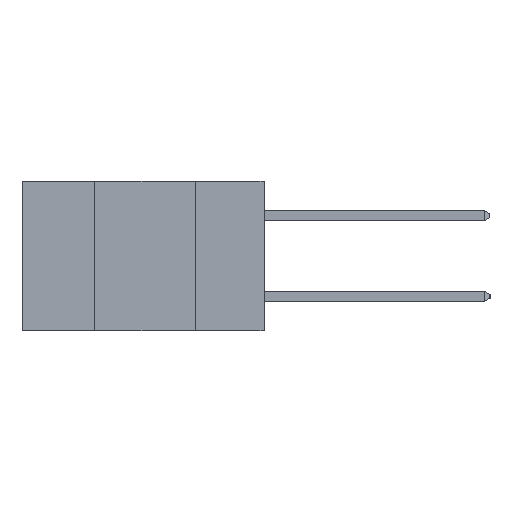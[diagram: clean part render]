
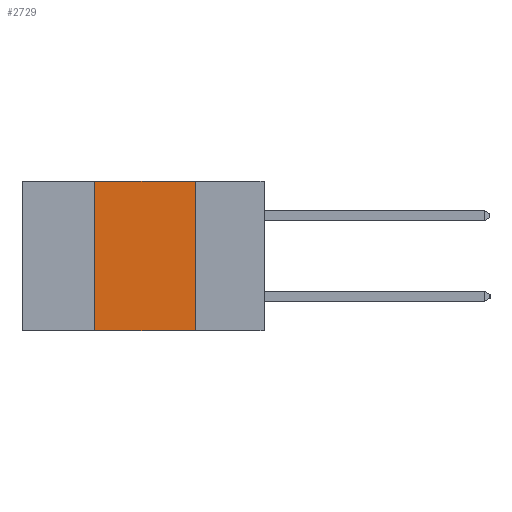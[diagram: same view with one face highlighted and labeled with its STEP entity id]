
A CAD part, left-side view. The second image highlights one B-rep face of the part: STEP entity #2729.
In plain terms, the highlighted planar face has unit normal (-1, 0, 0).
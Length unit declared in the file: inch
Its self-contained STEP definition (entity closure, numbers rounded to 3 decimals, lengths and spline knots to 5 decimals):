
#349 = DIRECTION ( 'NONE',  ( 0., -1., 0. ) ) ;
#1070 = EDGE_CURVE ( 'NONE', #13673, #6517, #11731, .T. ) ;
#2141 = ORIENTED_EDGE ( 'NONE', *, *, #1070, .F. ) ;
#2276 = CARTESIAN_POINT ( 'NONE',  ( 0., 0.17, -0.37 ) ) ;
#2729 = ADVANCED_FACE ( 'NONE', ( #12255 ), #10736, .F. ) ;
#3753 = LINE ( 'NONE', #13724, #12672 ) ;
#4193 = LINE ( 'NONE', #5024, #13782 ) ;
#4704 = EDGE_CURVE ( 'NONE', #12882, #13924, #4193, .T. ) ;
#4868 = VECTOR ( 'NONE', #349, 39.37008 ) ;
#4970 = DIRECTION ( 'NONE',  ( 0., -1., 0. ) ) ;
#5024 = CARTESIAN_POINT ( 'NONE',  ( 0., 0.6, -0.37 ) ) ;
#5704 = EDGE_CURVE ( 'NONE', #6517, #13924, #9442, .T. ) ;
#5843 = VECTOR ( 'NONE', #12835, 39.37008 ) ;
#6000 = CARTESIAN_POINT ( 'NONE',  ( 0., 0.42, -0.37 ) ) ;
#6517 = VERTEX_POINT ( 'NONE', #12447 ) ;
#7185 = ORIENTED_EDGE ( 'NONE', *, *, #5704, .F. ) ;
#7706 = CARTESIAN_POINT ( 'NONE',  ( 0., 0.42, 0. ) ) ;
#8224 = CARTESIAN_POINT ( 'NONE',  ( 0., 0.6, 0. ) ) ;
#9442 = LINE ( 'NONE', #12552, #5843 ) ;
#10076 = EDGE_LOOP ( 'NONE', ( #7185, #2141, #11559, #13896 ) ) ;
#10690 = CARTESIAN_POINT ( 'NONE',  ( 0., 0.6, 0. ) ) ;
#10736 = PLANE ( 'NONE',  #15499 ) ;
#10807 = DIRECTION ( 'NONE',  ( 1., 0., 0. ) ) ;
#10990 = DIRECTION ( 'NONE',  ( 0., 0., -1. ) ) ;
#11559 = ORIENTED_EDGE ( 'NONE', *, *, #14312, .F. ) ;
#11731 = LINE ( 'NONE', #8224, #4868 ) ;
#12255 = FACE_OUTER_BOUND ( 'NONE', #10076, .T. ) ;
#12447 = CARTESIAN_POINT ( 'NONE',  ( 0., 0.17, 0. ) ) ;
#12552 = CARTESIAN_POINT ( 'NONE',  ( 0., 0.17, -0.37 ) ) ;
#12672 = VECTOR ( 'NONE', #13659, 39.37008 ) ;
#12835 = DIRECTION ( 'NONE',  ( 0., 0., -1. ) ) ;
#12882 = VERTEX_POINT ( 'NONE', #6000 ) ;
#13659 = DIRECTION ( 'NONE',  ( 0., 0., 1. ) ) ;
#13673 = VERTEX_POINT ( 'NONE', #7706 ) ;
#13724 = CARTESIAN_POINT ( 'NONE',  ( 0., 0.42, -0.37 ) ) ;
#13782 = VECTOR ( 'NONE', #4970, 39.37008 ) ;
#13896 = ORIENTED_EDGE ( 'NONE', *, *, #4704, .T. ) ;
#13924 = VERTEX_POINT ( 'NONE', #2276 ) ;
#14312 = EDGE_CURVE ( 'NONE', #12882, #13673, #3753, .T. ) ;
#15499 = AXIS2_PLACEMENT_3D ( 'NONE', #10690, #10807, #10990 ) ;
